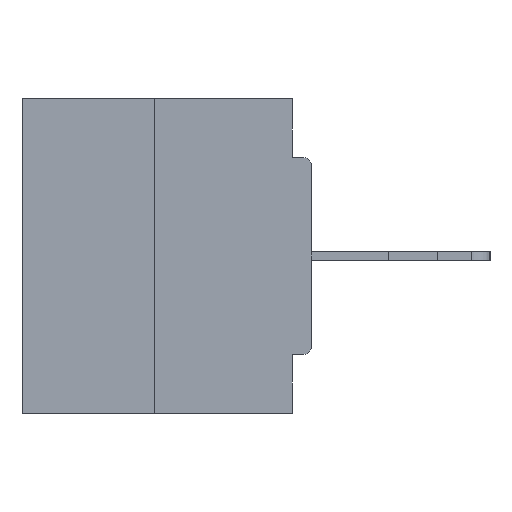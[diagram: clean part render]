
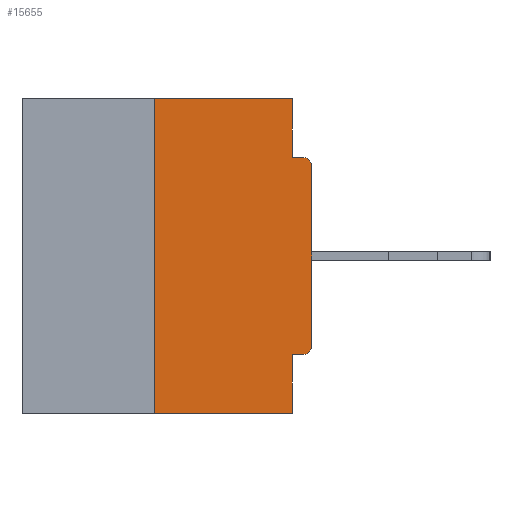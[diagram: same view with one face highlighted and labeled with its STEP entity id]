
A CAD part, left-side view. The second image highlights one B-rep face of the part: STEP entity #15655.
In plain terms, the highlighted planar face has unit normal (-1, 0, 0).
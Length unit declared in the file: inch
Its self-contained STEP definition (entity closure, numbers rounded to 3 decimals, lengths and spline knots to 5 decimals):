
#123 = AXIS2_PLACEMENT_3D ( 'NONE', #20558, #5375, #5048 ) ;
#355 = DIRECTION ( 'NONE',  ( 0., 0., -1. ) ) ;
#667 = VECTOR ( 'NONE', #17872, 39.37008 ) ;
#1381 = CARTESIAN_POINT ( 'NONE',  ( 0., 0., -0.4065 ) ) ;
#1447 = VERTEX_POINT ( 'NONE', #23924 ) ;
#1477 = VECTOR ( 'NONE', #7235, 39.37008 ) ;
#2003 = CARTESIAN_POINT ( 'NONE',  ( 0., 0.25, 0. ) ) ;
#2769 = DIRECTION ( 'NONE',  ( 0., -1., 0. ) ) ;
#3049 = DIRECTION ( 'NONE',  ( -1., 0., 0. ) ) ;
#4229 = FACE_OUTER_BOUND ( 'NONE', #9198, .T. ) ;
#4337 = EDGE_CURVE ( 'NONE', #6314, #21206, #24233, .T. ) ;
#4677 = VERTEX_POINT ( 'NONE', #23518 ) ;
#5048 = DIRECTION ( 'NONE',  ( 0., 0., -1. ) ) ;
#5375 = DIRECTION ( 'NONE',  ( 1., 0., 0. ) ) ;
#5658 = DIRECTION ( 'NONE',  ( -1., 0., 0. ) ) ;
#5833 = CARTESIAN_POINT ( 'NONE',  ( 0., 0.015, -0.3915 ) ) ;
#5890 = VERTEX_POINT ( 'NONE', #8179 ) ;
#5953 = ORIENTED_EDGE ( 'NONE', *, *, #4337, .T. ) ;
#6117 = LINE ( 'NONE', #1381, #21269 ) ;
#6314 = VERTEX_POINT ( 'NONE', #7820 ) ;
#6445 = VERTEX_POINT ( 'NONE', #28910 ) ;
#6523 = ORIENTED_EDGE ( 'NONE', *, *, #13175, .T. ) ;
#7235 = DIRECTION ( 'NONE',  ( 0., 0., 1. ) ) ;
#7314 = CARTESIAN_POINT ( 'NONE',  ( 0., 0.031, -0.0935 ) ) ;
#7576 = CARTESIAN_POINT ( 'NONE',  ( 0., 0.031, 0. ) ) ;
#7820 = CARTESIAN_POINT ( 'NONE',  ( 0., 0., -0.3915 ) ) ;
#8179 = CARTESIAN_POINT ( 'NONE',  ( 0., 0.031, -0.5 ) ) ;
#8381 = EDGE_CURVE ( 'NONE', #22108, #5890, #10444, .T. ) ;
#8490 = CIRCLE ( 'NONE', #22505, 0.015 ) ;
#8504 = ORIENTED_EDGE ( 'NONE', *, *, #8381, .F. ) ;
#8619 = VECTOR ( 'NONE', #2769, 39.37008 ) ;
#9198 = EDGE_LOOP ( 'NONE', ( #26415, #25672, #18197, #8504, #11755, #25353, #5953, #6523, #22716, #12992 ) ) ;
#10093 = LINE ( 'NONE', #7576, #667 ) ;
#10444 = LINE ( 'NONE', #17729, #14838 ) ;
#11070 = CARTESIAN_POINT ( 'NONE',  ( 0., 0., 0. ) ) ;
#11218 = DIRECTION ( 'NONE',  ( 0., 0., -1. ) ) ;
#11527 = VERTEX_POINT ( 'NONE', #24173 ) ;
#11729 = VECTOR ( 'NONE', #25289, 39.37008 ) ;
#11755 = ORIENTED_EDGE ( 'NONE', *, *, #19649, .F. ) ;
#12658 = DIRECTION ( 'NONE',  ( 0., 0., -1. ) ) ;
#12992 = ORIENTED_EDGE ( 'NONE', *, *, #15758, .F. ) ;
#13175 = EDGE_CURVE ( 'NONE', #21206, #1447, #26321, .T. ) ;
#13832 = VERTEX_POINT ( 'NONE', #7314 ) ;
#14000 = CARTESIAN_POINT ( 'NONE',  ( 0., 0.031, -0.4065 ) ) ;
#14514 = PLANE ( 'NONE',  #123 ) ;
#14632 = LINE ( 'NONE', #24907, #29947 ) ;
#14838 = VECTOR ( 'NONE', #12658, 39.37008 ) ;
#15655 = ADVANCED_FACE ( 'NONE', ( #4229 ), #14514, .F. ) ;
#15758 = EDGE_CURVE ( 'NONE', #11527, #13832, #10093, .T. ) ;
#17211 = LINE ( 'NONE', #30683, #11729 ) ;
#17729 = CARTESIAN_POINT ( 'NONE',  ( 0., 0.031, -0.5 ) ) ;
#17872 = DIRECTION ( 'NONE',  ( 0., 0., -1. ) ) ;
#18197 = ORIENTED_EDGE ( 'NONE', *, *, #28294, .T. ) ;
#19649 = EDGE_CURVE ( 'NONE', #24632, #22108, #6117, .T. ) ;
#20089 = VECTOR ( 'NONE', #21368, 39.37008 ) ;
#20558 = CARTESIAN_POINT ( 'NONE',  ( 0., 0.46, 0. ) ) ;
#20622 = EDGE_CURVE ( 'NONE', #6445, #11527, #14632, .T. ) ;
#20879 = CARTESIAN_POINT ( 'NONE',  ( 0., 0.015, -0.4065 ) ) ;
#21206 = VERTEX_POINT ( 'NONE', #22504 ) ;
#21269 = VECTOR ( 'NONE', #29563, 39.37008 ) ;
#21368 = DIRECTION ( 'NONE',  ( 0., 0., 1. ) ) ;
#22108 = VERTEX_POINT ( 'NONE', #14000 ) ;
#22299 = EDGE_CURVE ( 'NONE', #4677, #6445, #25114, .T. ) ;
#22504 = CARTESIAN_POINT ( 'NONE',  ( 0., 0., -0.1085 ) ) ;
#22505 = AXIS2_PLACEMENT_3D ( 'NONE', #5833, #5658, #11218 ) ;
#22548 = DIRECTION ( 'NONE',  ( 0., -1., 0. ) ) ;
#22716 = ORIENTED_EDGE ( 'NONE', *, *, #31277, .F. ) ;
#23518 = CARTESIAN_POINT ( 'NONE',  ( 0., 0.25, -0.5 ) ) ;
#23924 = CARTESIAN_POINT ( 'NONE',  ( 0., 0.015, -0.0935 ) ) ;
#24016 = EDGE_CURVE ( 'NONE', #24632, #6314, #8490, .T. ) ;
#24173 = CARTESIAN_POINT ( 'NONE',  ( 0., 0.031, 0. ) ) ;
#24233 = LINE ( 'NONE', #11070, #20089 ) ;
#24632 = VERTEX_POINT ( 'NONE', #20879 ) ;
#24907 = CARTESIAN_POINT ( 'NONE',  ( 0., 0.46, 0. ) ) ;
#25114 = LINE ( 'NONE', #2003, #1477 ) ;
#25289 = DIRECTION ( 'NONE',  ( 0., -1., 0. ) ) ;
#25353 = ORIENTED_EDGE ( 'NONE', *, *, #24016, .T. ) ;
#25672 = ORIENTED_EDGE ( 'NONE', *, *, #22299, .F. ) ;
#25876 = CARTESIAN_POINT ( 'NONE',  ( 0., 0., -0.0935 ) ) ;
#26150 = CARTESIAN_POINT ( 'NONE',  ( 0., 0.015, -0.1085 ) ) ;
#26321 = CIRCLE ( 'NONE', #29037, 0.015 ) ;
#26415 = ORIENTED_EDGE ( 'NONE', *, *, #20622, .F. ) ;
#28294 = EDGE_CURVE ( 'NONE', #4677, #5890, #17211, .T. ) ;
#28411 = LINE ( 'NONE', #25876, #8619 ) ;
#28910 = CARTESIAN_POINT ( 'NONE',  ( 0., 0.25, 0. ) ) ;
#29037 = AXIS2_PLACEMENT_3D ( 'NONE', #26150, #3049, #355 ) ;
#29563 = DIRECTION ( 'NONE',  ( 0., 1., 0. ) ) ;
#29947 = VECTOR ( 'NONE', #22548, 39.37008 ) ;
#30683 = CARTESIAN_POINT ( 'NONE',  ( 0., 0.46, -0.5 ) ) ;
#31277 = EDGE_CURVE ( 'NONE', #13832, #1447, #28411, .T. ) ;
